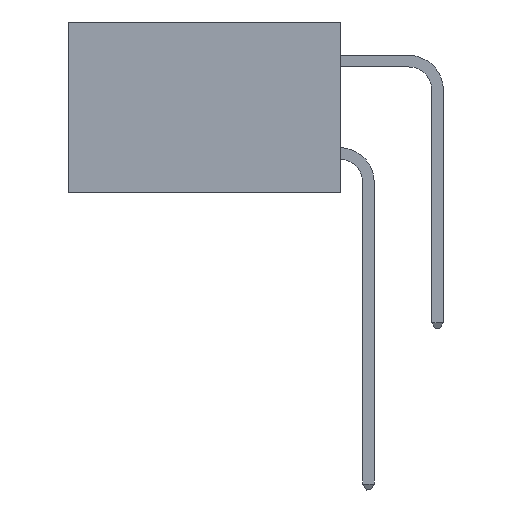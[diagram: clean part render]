
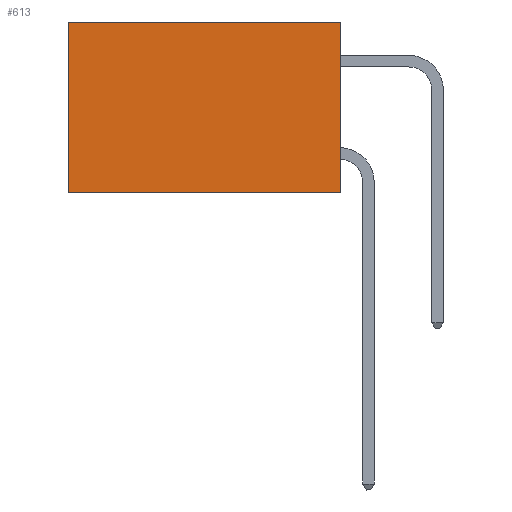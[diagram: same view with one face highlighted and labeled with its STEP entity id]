
A CAD part, left-side view. The second image highlights one B-rep face of the part: STEP entity #613.
In plain terms, the highlighted planar face has unit normal (-1, 0, 0).
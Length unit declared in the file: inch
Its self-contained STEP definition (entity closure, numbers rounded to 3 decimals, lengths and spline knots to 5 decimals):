
#613 = ADVANCED_FACE ( 'NONE', ( #21421 ), #18994, .F. ) ;
#1377 = DIRECTION ( 'NONE',  ( 0., 1., 0. ) ) ;
#2030 = VECTOR ( 'NONE', #15019, 39.37008 ) ;
#3693 = EDGE_LOOP ( 'NONE', ( #17405, #12233, #9789, #26651 ) ) ;
#3763 = VECTOR ( 'NONE', #1377, 39.37008 ) ;
#4048 = AXIS2_PLACEMENT_3D ( 'NONE', #16492, #24778, #27110 ) ;
#4943 = CARTESIAN_POINT ( 'NONE',  ( 0.277, 0., 0. ) ) ;
#5804 = CARTESIAN_POINT ( 'NONE',  ( 0.277, 0.59, -0.37 ) ) ;
#6387 = CARTESIAN_POINT ( 'NONE',  ( 0.277, 0., -0.37 ) ) ;
#7303 = CARTESIAN_POINT ( 'NONE',  ( 0.277, 0., -0.37 ) ) ;
#8768 = LINE ( 'NONE', #24875, #2030 ) ;
#9729 = LINE ( 'NONE', #6387, #3763 ) ;
#9789 = ORIENTED_EDGE ( 'NONE', *, *, #26413, .F. ) ;
#10904 = DIRECTION ( 'NONE',  ( 0., 0., -1. ) ) ;
#11618 = EDGE_CURVE ( 'NONE', #11666, #24188, #22021, .T. ) ;
#11666 = VERTEX_POINT ( 'NONE', #28654 ) ;
#12233 = ORIENTED_EDGE ( 'NONE', *, *, #30004, .F. ) ;
#14885 = LINE ( 'NONE', #31629, #28145 ) ;
#15019 = DIRECTION ( 'NONE',  ( 0., 0., -1. ) ) ;
#16492 = CARTESIAN_POINT ( 'NONE',  ( 0.277, 0., -0.37 ) ) ;
#16758 = DIRECTION ( 'NONE',  ( 0., 1., 0. ) ) ;
#17405 = ORIENTED_EDGE ( 'NONE', *, *, #11618, .T. ) ;
#18994 = PLANE ( 'NONE',  #4048 ) ;
#21421 = FACE_OUTER_BOUND ( 'NONE', #3693, .T. ) ;
#22021 = LINE ( 'NONE', #23459, #27814 ) ;
#23459 = CARTESIAN_POINT ( 'NONE',  ( 0.277, 0.59, -0.37 ) ) ;
#24188 = VERTEX_POINT ( 'NONE', #5804 ) ;
#24778 = DIRECTION ( 'NONE',  ( 1., 0., 0. ) ) ;
#24875 = CARTESIAN_POINT ( 'NONE',  ( 0.277, 0., -0.37 ) ) ;
#25145 = EDGE_CURVE ( 'NONE', #31638, #11666, #14885, .T. ) ;
#26403 = VERTEX_POINT ( 'NONE', #7303 ) ;
#26413 = EDGE_CURVE ( 'NONE', #31638, #26403, #8768, .T. ) ;
#26651 = ORIENTED_EDGE ( 'NONE', *, *, #25145, .T. ) ;
#27110 = DIRECTION ( 'NONE',  ( 0., 0., -1. ) ) ;
#27814 = VECTOR ( 'NONE', #10904, 39.37008 ) ;
#28145 = VECTOR ( 'NONE', #16758, 39.37008 ) ;
#28654 = CARTESIAN_POINT ( 'NONE',  ( 0.277, 0.59, 0. ) ) ;
#30004 = EDGE_CURVE ( 'NONE', #26403, #24188, #9729, .T. ) ;
#31629 = CARTESIAN_POINT ( 'NONE',  ( 0.277, 0., 0. ) ) ;
#31638 = VERTEX_POINT ( 'NONE', #4943 ) ;
